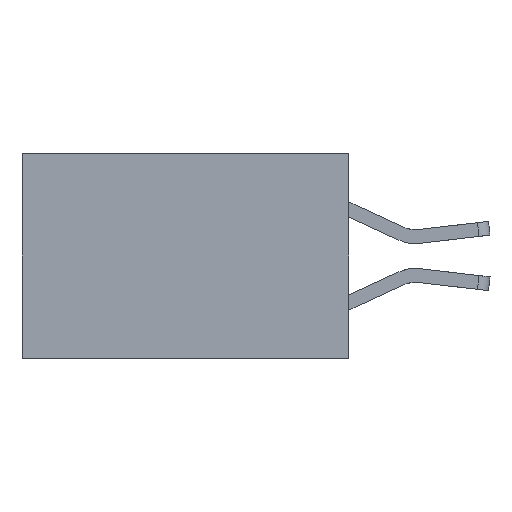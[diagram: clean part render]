
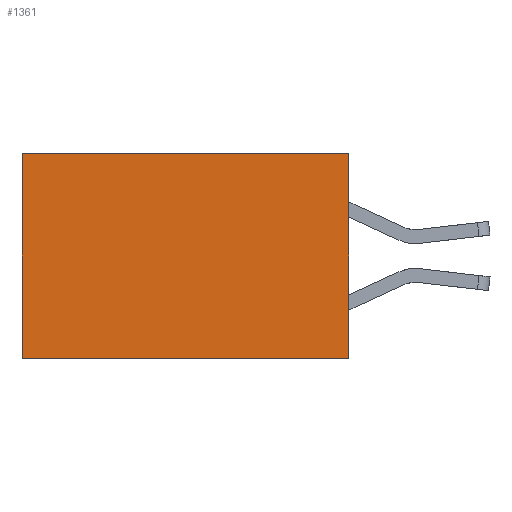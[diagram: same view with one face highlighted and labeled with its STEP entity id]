
A CAD part, left-side view. The second image highlights one B-rep face of the part: STEP entity #1361.
In plain terms, the highlighted planar face has unit normal (-1, 0, 0).
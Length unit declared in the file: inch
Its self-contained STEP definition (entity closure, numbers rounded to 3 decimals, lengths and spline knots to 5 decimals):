
#452 = VERTEX_POINT ( 'NONE', #8707 ) ;
#474 = VERTEX_POINT ( 'NONE', #1803 ) ;
#602 = LINE ( 'NONE', #8122, #8935 ) ;
#832 = VERTEX_POINT ( 'NONE', #4039 ) ;
#1144 = PLANE ( 'NONE',  #3243 ) ;
#1361 = ADVANCED_FACE ( 'NONE', ( #3530 ), #1144, .F. ) ;
#1520 = ORIENTED_EDGE ( 'NONE', *, *, #5616, .T. ) ;
#1803 = CARTESIAN_POINT ( 'NONE',  ( 0.277, 0., -0.37 ) ) ;
#2696 = CARTESIAN_POINT ( 'NONE',  ( 0.277, 0., -0.37 ) ) ;
#2921 = DIRECTION ( 'NONE',  ( 0., 0., -1. ) ) ;
#2925 = CARTESIAN_POINT ( 'NONE',  ( 0.277, 0.59, -0.37 ) ) ;
#3104 = CARTESIAN_POINT ( 'NONE',  ( 0.277, 0.59, -0.37 ) ) ;
#3127 = DIRECTION ( 'NONE',  ( 1., 0., 0. ) ) ;
#3193 = EDGE_LOOP ( 'NONE', ( #1520, #5942, #7906, #4021 ) ) ;
#3233 = EDGE_CURVE ( 'NONE', #832, #452, #8197, .T. ) ;
#3243 = AXIS2_PLACEMENT_3D ( 'NONE', #2696, #3127, #7658 ) ;
#3492 = DIRECTION ( 'NONE',  ( 0., 1., 0. ) ) ;
#3530 = FACE_OUTER_BOUND ( 'NONE', #3193, .T. ) ;
#3826 = VECTOR ( 'NONE', #2921, 39.37008 ) ;
#4021 = ORIENTED_EDGE ( 'NONE', *, *, #3233, .T. ) ;
#4039 = CARTESIAN_POINT ( 'NONE',  ( 0.277, 0., 0. ) ) ;
#4134 = VECTOR ( 'NONE', #7905, 39.37008 ) ;
#4267 = EDGE_CURVE ( 'NONE', #832, #474, #6441, .T. ) ;
#4711 = DIRECTION ( 'NONE',  ( 0., 0., -1. ) ) ;
#4820 = CARTESIAN_POINT ( 'NONE',  ( 0.277, 0., -0.37 ) ) ;
#5251 = EDGE_CURVE ( 'NONE', #474, #7335, #602, .T. ) ;
#5616 = EDGE_CURVE ( 'NONE', #452, #7335, #8151, .T. ) ;
#5942 = ORIENTED_EDGE ( 'NONE', *, *, #5251, .F. ) ;
#6441 = LINE ( 'NONE', #4820, #9317 ) ;
#7335 = VERTEX_POINT ( 'NONE', #2925 ) ;
#7658 = DIRECTION ( 'NONE',  ( 0., 0., -1. ) ) ;
#7905 = DIRECTION ( 'NONE',  ( 0., 1., 0. ) ) ;
#7906 = ORIENTED_EDGE ( 'NONE', *, *, #4267, .F. ) ;
#7953 = CARTESIAN_POINT ( 'NONE',  ( 0.277, 0., 0. ) ) ;
#8122 = CARTESIAN_POINT ( 'NONE',  ( 0.277, 0., -0.37 ) ) ;
#8151 = LINE ( 'NONE', #3104, #3826 ) ;
#8197 = LINE ( 'NONE', #7953, #4134 ) ;
#8707 = CARTESIAN_POINT ( 'NONE',  ( 0.277, 0.59, 0. ) ) ;
#8935 = VECTOR ( 'NONE', #3492, 39.37008 ) ;
#9317 = VECTOR ( 'NONE', #4711, 39.37008 ) ;
